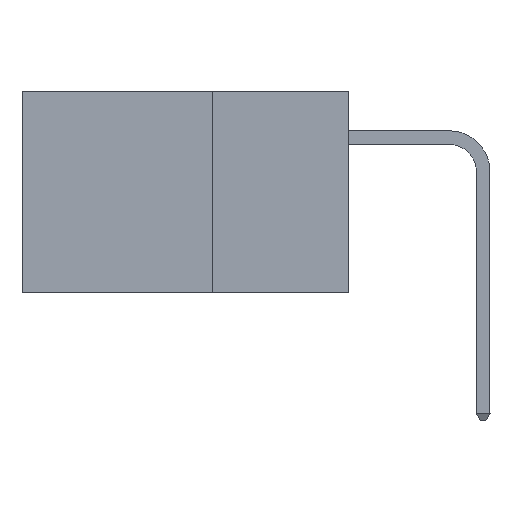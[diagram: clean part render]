
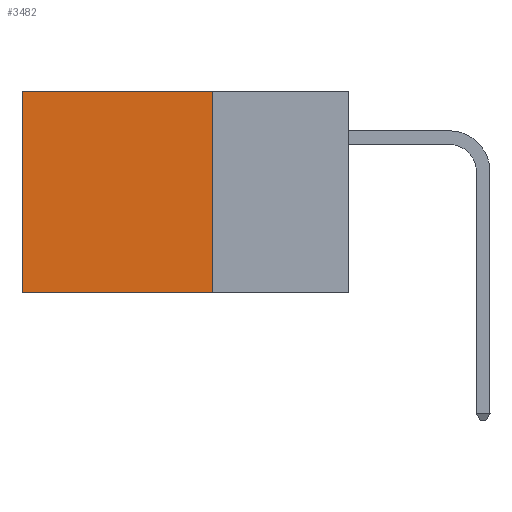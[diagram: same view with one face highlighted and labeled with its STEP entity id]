
A CAD part, left-side view. The second image highlights one B-rep face of the part: STEP entity #3482.
In plain terms, the highlighted planar face has unit normal (-1, 0, 0).
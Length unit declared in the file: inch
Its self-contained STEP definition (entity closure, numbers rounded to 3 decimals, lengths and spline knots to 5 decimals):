
#1168 = EDGE_LOOP ( 'NONE', ( #6074, #16786, #46423, #5559 ) ) ;
#3482 = ADVANCED_FACE ( 'NONE', ( #6240 ), #31954, .F. ) ;
#4383 = CARTESIAN_POINT ( 'NONE',  ( 0.2875, 0.25, 0. ) ) ;
#5559 = ORIENTED_EDGE ( 'NONE', *, *, #41693, .T. ) ;
#5913 = VERTEX_POINT ( 'NONE', #15475 ) ;
#6074 = ORIENTED_EDGE ( 'NONE', *, *, #8078, .T. ) ;
#6240 = FACE_OUTER_BOUND ( 'NONE', #1168, .T. ) ;
#8078 = EDGE_CURVE ( 'NONE', #26022, #5913, #35365, .T. ) ;
#8927 = VERTEX_POINT ( 'NONE', #38039 ) ;
#14750 = CARTESIAN_POINT ( 'NONE',  ( 0.2875, 0.25, -0.37 ) ) ;
#15095 = VERTEX_POINT ( 'NONE', #21785 ) ;
#15475 = CARTESIAN_POINT ( 'NONE',  ( 0.2875, 0.6, -0.37 ) ) ;
#16786 = ORIENTED_EDGE ( 'NONE', *, *, #29426, .F. ) ;
#17762 = VECTOR ( 'NONE', #45970, 39.37008 ) ;
#18332 = VECTOR ( 'NONE', #34512, 39.37008 ) ;
#20054 = VECTOR ( 'NONE', #39700, 39.37008 ) ;
#21319 = CARTESIAN_POINT ( 'NONE',  ( 0.2875, 0.25, 0. ) ) ;
#21430 = LINE ( 'NONE', #14750, #40040 ) ;
#21731 = EDGE_CURVE ( 'NONE', #8927, #15095, #41911, .T. ) ;
#21785 = CARTESIAN_POINT ( 'NONE',  ( 0.2875, 0.25, -0.37 ) ) ;
#26022 = VERTEX_POINT ( 'NONE', #46732 ) ;
#28122 = LINE ( 'NONE', #42675, #20054 ) ;
#28487 = DIRECTION ( 'NONE',  ( 0., 0., -1. ) ) ;
#29426 = EDGE_CURVE ( 'NONE', #15095, #5913, #21430, .T. ) ;
#30928 = CARTESIAN_POINT ( 'NONE',  ( 0.2875, 0.6, 0. ) ) ;
#31954 = PLANE ( 'NONE',  #47058 ) ;
#34512 = DIRECTION ( 'NONE',  ( 0., 0., -1. ) ) ;
#35365 = LINE ( 'NONE', #30928, #17762 ) ;
#36350 = DIRECTION ( 'NONE',  ( 1., 0., 0. ) ) ;
#36707 = DIRECTION ( 'NONE',  ( 0., 1., 0. ) ) ;
#38039 = CARTESIAN_POINT ( 'NONE',  ( 0.2875, 0.25, 0. ) ) ;
#39700 = DIRECTION ( 'NONE',  ( 0., 1., 0. ) ) ;
#40040 = VECTOR ( 'NONE', #36707, 39.37008 ) ;
#41693 = EDGE_CURVE ( 'NONE', #8927, #26022, #28122, .T. ) ;
#41911 = LINE ( 'NONE', #4383, #18332 ) ;
#42675 = CARTESIAN_POINT ( 'NONE',  ( 0.2875, 0.25, 0. ) ) ;
#45970 = DIRECTION ( 'NONE',  ( 0., 0., -1. ) ) ;
#46423 = ORIENTED_EDGE ( 'NONE', *, *, #21731, .F. ) ;
#46732 = CARTESIAN_POINT ( 'NONE',  ( 0.2875, 0.6, 0. ) ) ;
#47058 = AXIS2_PLACEMENT_3D ( 'NONE', #21319, #36350, #28487 ) ;
